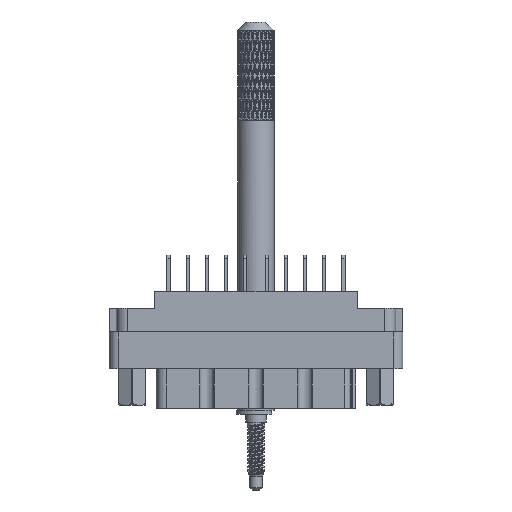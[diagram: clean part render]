
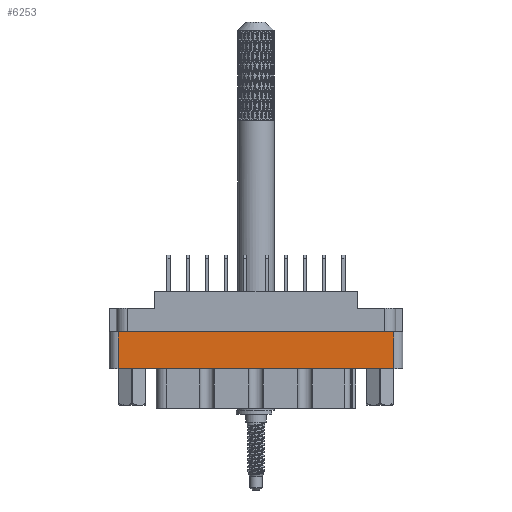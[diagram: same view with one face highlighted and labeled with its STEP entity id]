
A CAD part, front view. The second image highlights one B-rep face of the part: STEP entity #6253.
In plain terms, the highlighted planar face has unit normal (0, -1, 0).
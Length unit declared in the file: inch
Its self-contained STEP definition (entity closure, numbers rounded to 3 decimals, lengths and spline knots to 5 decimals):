
#3030 = PLANE ( 'NONE',  #36645 ) ;
#6253 = ADVANCED_FACE ( 'NONE', ( #90174 ), #3030, .T. ) ;
#7036 = LINE ( 'NONE', #85014, #49724 ) ;
#7144 = VERTEX_POINT ( 'NONE', #24791 ) ;
#7517 = LINE ( 'NONE', #34480, #58109 ) ;
#10173 = EDGE_CURVE ( 'NONE', #33014, #7144, #7036, .T. ) ;
#13234 = CARTESIAN_POINT ( 'NONE',  ( -0.938, -0.438, -0.277 ) ) ;
#14405 = ORIENTED_EDGE ( 'NONE', *, *, #10173, .F. ) ;
#24791 = CARTESIAN_POINT ( 'NONE',  ( -0.938, -0.438, -0.529 ) ) ;
#26659 = EDGE_CURVE ( 'NONE', #65162, #7144, #7517, .T. ) ;
#27458 = ORIENTED_EDGE ( 'NONE', *, *, #107657, .T. ) ;
#33014 = VERTEX_POINT ( 'NONE', #39619 ) ;
#34480 = CARTESIAN_POINT ( 'NONE',  ( -0.938, -0.438, -0.798 ) ) ;
#36645 = AXIS2_PLACEMENT_3D ( 'NONE', #70764, #80429, #80989 ) ;
#39619 = CARTESIAN_POINT ( 'NONE',  ( 0.938, -0.438, -0.529 ) ) ;
#40360 = VERTEX_POINT ( 'NONE', #51209 ) ;
#47524 = CARTESIAN_POINT ( 'NONE',  ( 0.938, -0.438, -0.798 ) ) ;
#49724 = VECTOR ( 'NONE', #58091, 39.37008 ) ;
#50717 = DIRECTION ( 'NONE',  ( 1., 0., 0. ) ) ;
#51209 = CARTESIAN_POINT ( 'NONE',  ( 0.938, -0.438, -0.277 ) ) ;
#52810 = DIRECTION ( 'NONE',  ( 0., 0., -1. ) ) ;
#55566 = LINE ( 'NONE', #47524, #81454 ) ;
#58091 = DIRECTION ( 'NONE',  ( -1., 0., 0. ) ) ;
#58109 = VECTOR ( 'NONE', #52810, 39.37008 ) ;
#62416 = EDGE_LOOP ( 'NONE', ( #75081, #104115, #14405, #27458 ) ) ;
#63610 = DIRECTION ( 'NONE',  ( 0., 0., 1. ) ) ;
#65162 = VERTEX_POINT ( 'NONE', #13234 ) ;
#70764 = CARTESIAN_POINT ( 'NONE',  ( -1., -0.438, -0.798 ) ) ;
#73880 = VECTOR ( 'NONE', #50717, 39.37008 ) ;
#75081 = ORIENTED_EDGE ( 'NONE', *, *, #81578, .F. ) ;
#80429 = DIRECTION ( 'NONE',  ( 0., -1., 0. ) ) ;
#80989 = DIRECTION ( 'NONE',  ( 0., 0., -1. ) ) ;
#81454 = VECTOR ( 'NONE', #63610, 39.37008 ) ;
#81578 = EDGE_CURVE ( 'NONE', #65162, #40360, #105098, .T. ) ;
#85014 = CARTESIAN_POINT ( 'NONE',  ( 0., -0.438, -0.529 ) ) ;
#86235 = CARTESIAN_POINT ( 'NONE',  ( 0., -0.438, -0.277 ) ) ;
#90174 = FACE_OUTER_BOUND ( 'NONE', #62416, .T. ) ;
#104115 = ORIENTED_EDGE ( 'NONE', *, *, #26659, .T. ) ;
#105098 = LINE ( 'NONE', #86235, #73880 ) ;
#107657 = EDGE_CURVE ( 'NONE', #33014, #40360, #55566, .T. ) ;
